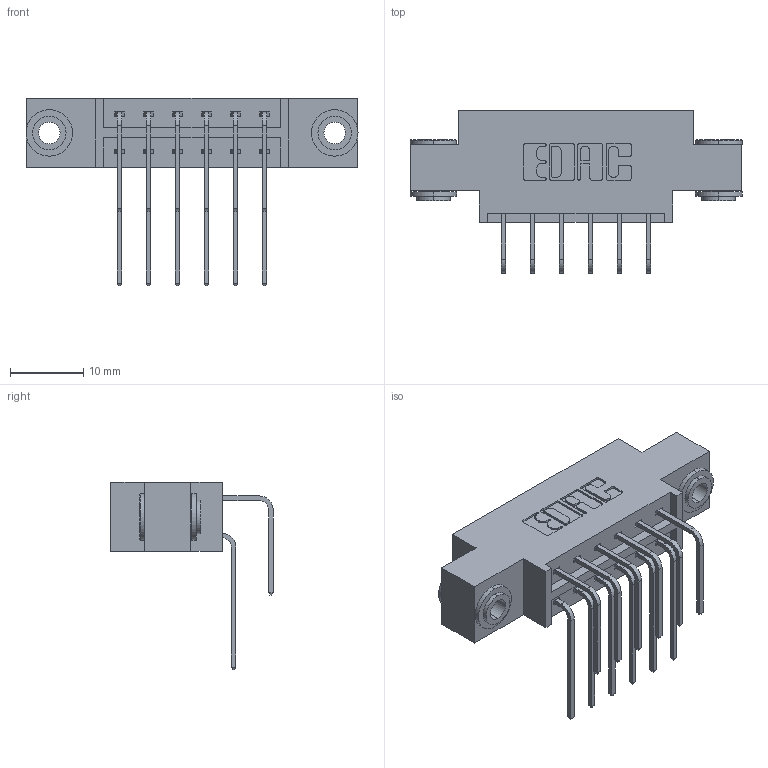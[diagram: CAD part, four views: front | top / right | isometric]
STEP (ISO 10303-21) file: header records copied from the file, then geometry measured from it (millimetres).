
FILE_DESCRIPTION (( 'STEP AP203' ), '1' );
FILE_NAME ('833-012-558-803.STEP', '2020-05-30T22:57:42', ( '' ), ( '' ), 'SwSTEP 2.0', 'SolidWorks 2020', '' );
FILE_SCHEMA (( 'CONFIG_CONTROL_DESIGN' ));
Length unit declared in the file: inch
Products named in the file (5): 345-250-002_345-250-002-102; 833 Part_Offset - .156 Dia - TH; 345-292-001_558 Tail - 2; 345-292-001_558 559 Tail - 1; 833-012-558-803
Assembly tree (15 placements, depth 2):
  833-012-558-803
    833 Part_Offset - .156 Dia - TH
    345-292-001_558 559 Tail - 1  x6
    345-292-001_558 Tail - 2  x6
    345-250-002_345-250-002-102  x2
Bounding box: 45.31 x 22.17 x 25.53 mm (x, y, z)
Volume: 4150.4 mm3; surface area: 5306.5 mm2
Topology: 15 solids, 15 shells, 804 faces, 2331 edges, 1534 vertices
Faces by surface type: plane 540, cylinder 256, cone 8
Entity records: 11082 total; most frequent: CARTESIAN_POINT 1908, ORIENTED_EDGE 1786, DIRECTION 1707, EDGE_CURVE 893, LINE 701, VECTOR 701, VERTEX_POINT 590, AXIS2_PLACEMENT_3D 503
